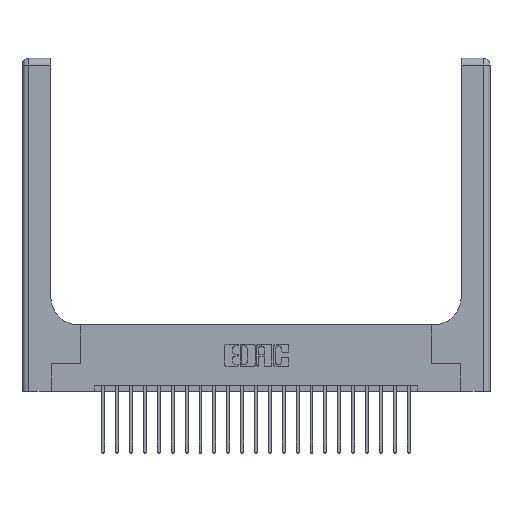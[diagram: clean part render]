
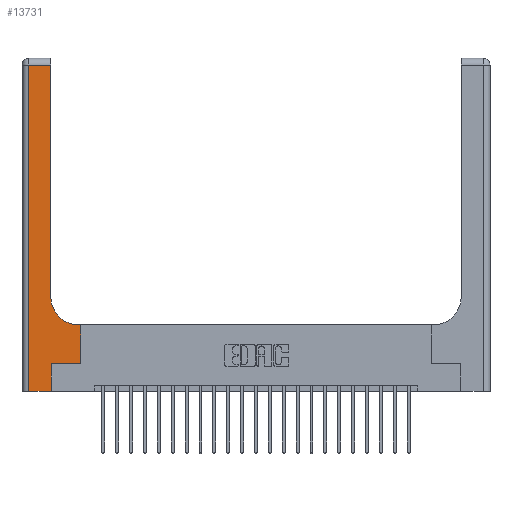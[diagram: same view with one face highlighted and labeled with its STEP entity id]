
A CAD part, top view. The second image highlights one B-rep face of the part: STEP entity #13731.
In plain terms, the highlighted planar face has unit normal (0, 0, 1).
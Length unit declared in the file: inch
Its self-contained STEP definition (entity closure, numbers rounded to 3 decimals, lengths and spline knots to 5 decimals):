
#231 = CARTESIAN_POINT ( 'NONE',  ( 0.06, 3., 0.37 ) ) ;
#503 = DIRECTION ( 'NONE',  ( 1., 0., 0. ) ) ;
#536 = LINE ( 'NONE', #9348, #18442 ) ;
#671 = VERTEX_POINT ( 'NONE', #12263 ) ;
#1139 = ORIENTED_EDGE ( 'NONE', *, *, #15234, .T. ) ;
#1895 = DIRECTION ( 'NONE',  ( -1., 0., 0. ) ) ;
#2104 = EDGE_CURVE ( 'NONE', #13748, #19393, #21828, .T. ) ;
#2271 = VERTEX_POINT ( 'NONE', #11826 ) ;
#2431 = CARTESIAN_POINT ( 'NONE',  ( 0.265, 0.25, 0.37 ) ) ;
#3793 = CARTESIAN_POINT ( 'NONE',  ( 0., 2.94, 0.37 ) ) ;
#4164 = DIRECTION ( 'NONE',  ( 0., 1., 0. ) ) ;
#4254 = EDGE_CURVE ( 'NONE', #11918, #671, #6020, .T. ) ;
#4370 = VERTEX_POINT ( 'NONE', #12962 ) ;
#4780 = EDGE_CURVE ( 'NONE', #8071, #11918, #17983, .T. ) ;
#4871 = EDGE_CURVE ( 'NONE', #20890, #2271, #5870, .T. ) ;
#5870 = LINE ( 'NONE', #6333, #8534 ) ;
#6020 = LINE ( 'NONE', #20224, #20907 ) ;
#6326 = CARTESIAN_POINT ( 'NONE',  ( 0.06, 2.94, 0.37 ) ) ;
#6333 = CARTESIAN_POINT ( 'NONE',  ( 0.26, 3., 0.37 ) ) ;
#7483 = CIRCLE ( 'NONE', #10481, 0.25 ) ;
#7829 = DIRECTION ( 'NONE',  ( -1., 0., 0. ) ) ;
#8071 = VERTEX_POINT ( 'NONE', #6326 ) ;
#8534 = VECTOR ( 'NONE', #22309, 39.37008 ) ;
#9348 = CARTESIAN_POINT ( 'NONE',  ( 0.528, 0.25, 0.37 ) ) ;
#9432 = VECTOR ( 'NONE', #1895, 39.37008 ) ;
#9489 = DIRECTION ( 'NONE',  ( 0., 0., -1. ) ) ;
#9587 = CARTESIAN_POINT ( 'NONE',  ( 0.265, 0.25, 0.37 ) ) ;
#10130 = AXIS2_PLACEMENT_3D ( 'NONE', #14668, #9489, #7829 ) ;
#10295 = CARTESIAN_POINT ( 'NONE',  ( 0.528, 0.25, 0.37 ) ) ;
#10481 = AXIS2_PLACEMENT_3D ( 'NONE', #20779, #13737, #13637 ) ;
#10806 = CARTESIAN_POINT ( 'NONE',  ( 0.51, 0.6, 0.37 ) ) ;
#10813 = LINE ( 'NONE', #14463, #9432 ) ;
#11175 = VECTOR ( 'NONE', #14702, 39.37008 ) ;
#11261 = FACE_OUTER_BOUND ( 'NONE', #13049, .T. ) ;
#11826 = CARTESIAN_POINT ( 'NONE',  ( 0.26, 2.94, 0.37 ) ) ;
#11860 = ORIENTED_EDGE ( 'NONE', *, *, #4871, .T. ) ;
#11918 = VERTEX_POINT ( 'NONE', #18067 ) ;
#12263 = CARTESIAN_POINT ( 'NONE',  ( 0.265, 0., 0.37 ) ) ;
#12745 = DIRECTION ( 'NONE',  ( -1., 0., 0. ) ) ;
#12962 = CARTESIAN_POINT ( 'NONE',  ( 0.528, 0.6, 0.37 ) ) ;
#13049 = EDGE_LOOP ( 'NONE', ( #11860, #16920, #16957, #19313, #19654, #19215, #1139, #14414, #19634 ) ) ;
#13620 = EDGE_CURVE ( 'NONE', #671, #13748, #15721, .T. ) ;
#13637 = DIRECTION ( 'NONE',  ( 1., 0., 0. ) ) ;
#13731 = ADVANCED_FACE ( 'NONE', ( #11261 ), #18419, .F. ) ;
#13737 = DIRECTION ( 'NONE',  ( 0., 0., -1. ) ) ;
#13748 = VERTEX_POINT ( 'NONE', #2431 ) ;
#14312 = CARTESIAN_POINT ( 'NONE',  ( 0.265, 0., 0.37 ) ) ;
#14414 = ORIENTED_EDGE ( 'NONE', *, *, #23142, .T. ) ;
#14463 = CARTESIAN_POINT ( 'NONE',  ( 0.26, 0.6, 0.37 ) ) ;
#14546 = CARTESIAN_POINT ( 'NONE',  ( 0.26, 0.85, 0.37 ) ) ;
#14668 = CARTESIAN_POINT ( 'NONE',  ( 0., 3., 0.37 ) ) ;
#14702 = DIRECTION ( 'NONE',  ( 0., -1., 0. ) ) ;
#15234 = EDGE_CURVE ( 'NONE', #19393, #4370, #536, .T. ) ;
#15721 = LINE ( 'NONE', #14312, #18756 ) ;
#16920 = ORIENTED_EDGE ( 'NONE', *, *, #16985, .T. ) ;
#16957 = ORIENTED_EDGE ( 'NONE', *, *, #4780, .T. ) ;
#16985 = EDGE_CURVE ( 'NONE', #2271, #8071, #20115, .T. ) ;
#17331 = VERTEX_POINT ( 'NONE', #10806 ) ;
#17461 = VECTOR ( 'NONE', #18288, 39.37008 ) ;
#17720 = DIRECTION ( 'NONE',  ( 0., 1., 0. ) ) ;
#17752 = VECTOR ( 'NONE', #12745, 39.37008 ) ;
#17983 = LINE ( 'NONE', #231, #11175 ) ;
#18067 = CARTESIAN_POINT ( 'NONE',  ( 0.06, 0., 0.37 ) ) ;
#18288 = DIRECTION ( 'NONE',  ( 1., 0., 0. ) ) ;
#18419 = PLANE ( 'NONE',  #10130 ) ;
#18442 = VECTOR ( 'NONE', #4164, 39.37008 ) ;
#18756 = VECTOR ( 'NONE', #17720, 39.37008 ) ;
#19215 = ORIENTED_EDGE ( 'NONE', *, *, #2104, .T. ) ;
#19313 = ORIENTED_EDGE ( 'NONE', *, *, #4254, .T. ) ;
#19393 = VERTEX_POINT ( 'NONE', #10295 ) ;
#19634 = ORIENTED_EDGE ( 'NONE', *, *, #20709, .T. ) ;
#19654 = ORIENTED_EDGE ( 'NONE', *, *, #13620, .T. ) ;
#20115 = LINE ( 'NONE', #3793, #17752 ) ;
#20224 = CARTESIAN_POINT ( 'NONE',  ( 0., 0., 0.37 ) ) ;
#20709 = EDGE_CURVE ( 'NONE', #17331, #20890, #7483, .T. ) ;
#20779 = CARTESIAN_POINT ( 'NONE',  ( 0.51, 0.85, 0.37 ) ) ;
#20890 = VERTEX_POINT ( 'NONE', #14546 ) ;
#20907 = VECTOR ( 'NONE', #503, 39.37008 ) ;
#21828 = LINE ( 'NONE', #9587, #17461 ) ;
#22309 = DIRECTION ( 'NONE',  ( 0., 1., 0. ) ) ;
#23142 = EDGE_CURVE ( 'NONE', #4370, #17331, #10813, .T. ) ;
